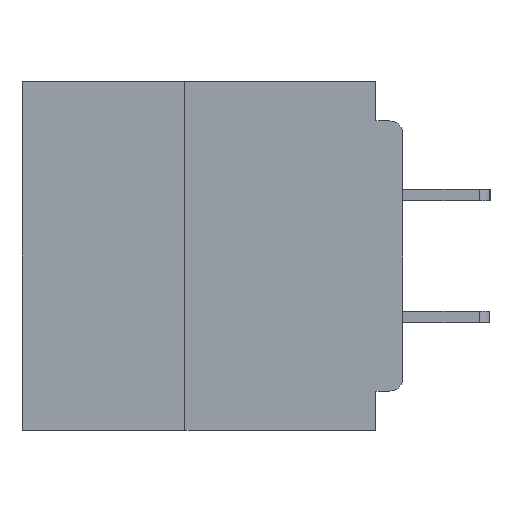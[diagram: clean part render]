
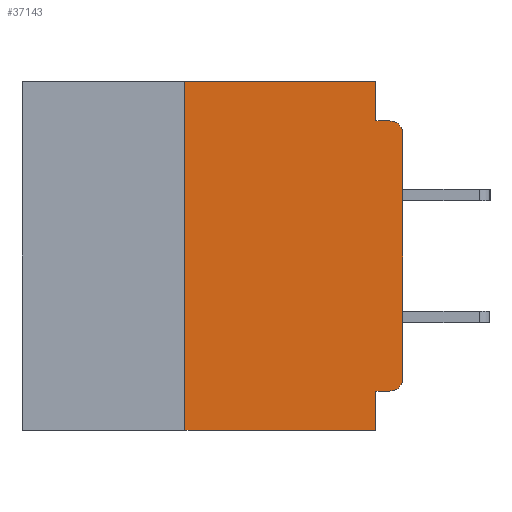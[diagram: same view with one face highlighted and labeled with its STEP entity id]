
A CAD part, left-side view. The second image highlights one B-rep face of the part: STEP entity #37143.
In plain terms, the highlighted planar face has unit normal (-1, 0, 0).
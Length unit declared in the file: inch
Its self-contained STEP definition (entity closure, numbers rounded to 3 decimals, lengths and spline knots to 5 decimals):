
#194 = CARTESIAN_POINT ( 'NONE',  ( 0., 0., -0.34 ) ) ;
#1139 = DIRECTION ( 'NONE',  ( 0., 0., 1. ) ) ;
#1416 = CARTESIAN_POINT ( 'NONE',  ( 0., 0.437, -0.4 ) ) ;
#1849 = DIRECTION ( 'NONE',  ( 0., 0., -1. ) ) ;
#1980 = CARTESIAN_POINT ( 'NONE',  ( 0., 0.031, -0.4 ) ) ;
#2558 = DIRECTION ( 'NONE',  ( 0., 0., -1. ) ) ;
#3075 = VERTEX_POINT ( 'NONE', #43019 ) ;
#3328 = EDGE_CURVE ( 'NONE', #17526, #16459, #58181, .T. ) ;
#5080 = AXIS2_PLACEMENT_3D ( 'NONE', #41207, #13744, #45778 ) ;
#6140 = LINE ( 'NONE', #47722, #52141 ) ;
#6951 = CARTESIAN_POINT ( 'NONE',  ( 0., 0.031, 0. ) ) ;
#7068 = PLANE ( 'NONE',  #7717 ) ;
#7717 = AXIS2_PLACEMENT_3D ( 'NONE', #52818, #30285, #2558 ) ;
#11805 = VECTOR ( 'NONE', #40488, 39.37008 ) ;
#12068 = DIRECTION ( 'NONE',  ( -1., 0., 0. ) ) ;
#13032 = VERTEX_POINT ( 'NONE', #49838 ) ;
#13688 = LINE ( 'NONE', #22514, #33827 ) ;
#13744 = DIRECTION ( 'NONE',  ( -1., 0., 0. ) ) ;
#14182 = EDGE_CURVE ( 'NONE', #31642, #31044, #6140, .T. ) ;
#15080 = VECTOR ( 'NONE', #39627, 39.37008 ) ;
#16413 = LINE ( 'NONE', #1416, #27245 ) ;
#16459 = VERTEX_POINT ( 'NONE', #194 ) ;
#17526 = VERTEX_POINT ( 'NONE', #19386 ) ;
#17550 = VERTEX_POINT ( 'NONE', #33222 ) ;
#17689 = CARTESIAN_POINT ( 'NONE',  ( 0., 0., 0. ) ) ;
#18527 = VECTOR ( 'NONE', #1139, 39.37008 ) ;
#19386 = CARTESIAN_POINT ( 'NONE',  ( 0., 0.015, -0.355 ) ) ;
#20598 = DIRECTION ( 'NONE',  ( 0., 1., 0. ) ) ;
#22514 = CARTESIAN_POINT ( 'NONE',  ( 0., 0.031, 0. ) ) ;
#23366 = EDGE_CURVE ( 'NONE', #48259, #13032, #50401, .T. ) ;
#23539 = CARTESIAN_POINT ( 'NONE',  ( 0., 0.25, 0. ) ) ;
#23822 = ORIENTED_EDGE ( 'NONE', *, *, #3328, .T. ) ;
#24265 = CARTESIAN_POINT ( 'NONE',  ( 0., 0.25, -0.4 ) ) ;
#24963 = ORIENTED_EDGE ( 'NONE', *, *, #56077, .F. ) ;
#25445 = VERTEX_POINT ( 'NONE', #23539 ) ;
#25500 = EDGE_CURVE ( 'NONE', #17550, #13032, #26323, .T. ) ;
#26066 = ORIENTED_EDGE ( 'NONE', *, *, #56413, .F. ) ;
#26150 = EDGE_CURVE ( 'NONE', #16459, #48259, #34818, .T. ) ;
#26323 = LINE ( 'NONE', #42097, #35615 ) ;
#27039 = ORIENTED_EDGE ( 'NONE', *, *, #53237, .F. ) ;
#27245 = VECTOR ( 'NONE', #51910, 39.37008 ) ;
#27362 = LINE ( 'NONE', #35068, #15080 ) ;
#28118 = CARTESIAN_POINT ( 'NONE',  ( 0., 0., -0.06 ) ) ;
#28963 = ORIENTED_EDGE ( 'NONE', *, *, #36351, .T. ) ;
#29972 = FACE_OUTER_BOUND ( 'NONE', #37342, .T. ) ;
#30285 = DIRECTION ( 'NONE',  ( 1., 0., 0. ) ) ;
#31044 = VERTEX_POINT ( 'NONE', #1980 ) ;
#31642 = VERTEX_POINT ( 'NONE', #51182 ) ;
#31909 = DIRECTION ( 'NONE',  ( 0., 0., -1. ) ) ;
#32464 = LINE ( 'NONE', #43373, #53875 ) ;
#33222 = CARTESIAN_POINT ( 'NONE',  ( 0., 0.031, -0.045 ) ) ;
#33699 = ORIENTED_EDGE ( 'NONE', *, *, #26150, .T. ) ;
#33827 = VECTOR ( 'NONE', #31909, 39.37008 ) ;
#34818 = LINE ( 'NONE', #17689, #11805 ) ;
#35068 = CARTESIAN_POINT ( 'NONE',  ( 0., 0.437, 0. ) ) ;
#35615 = VECTOR ( 'NONE', #46691, 39.37008 ) ;
#36351 = EDGE_CURVE ( 'NONE', #3075, #31044, #16413, .T. ) ;
#36957 = EDGE_CURVE ( 'NONE', #3075, #25445, #42836, .T. ) ;
#37143 = ADVANCED_FACE ( 'NONE', ( #29972 ), #7068, .F. ) ;
#37342 = EDGE_LOOP ( 'NONE', ( #33699, #42407, #50596, #24963, #26066, #41980, #28963, #55460, #27039, #23822 ) ) ;
#39539 = CARTESIAN_POINT ( 'NONE',  ( 0., 0.015, -0.06 ) ) ;
#39627 = DIRECTION ( 'NONE',  ( 0., -1., 0. ) ) ;
#40488 = DIRECTION ( 'NONE',  ( 0., 0., 1. ) ) ;
#41207 = CARTESIAN_POINT ( 'NONE',  ( 0., 0.015, -0.34 ) ) ;
#41980 = ORIENTED_EDGE ( 'NONE', *, *, #36957, .F. ) ;
#42097 = CARTESIAN_POINT ( 'NONE',  ( 0., 0., -0.045 ) ) ;
#42407 = ORIENTED_EDGE ( 'NONE', *, *, #23366, .T. ) ;
#42836 = LINE ( 'NONE', #24265, #18527 ) ;
#43019 = CARTESIAN_POINT ( 'NONE',  ( 0., 0.25, -0.4 ) ) ;
#43373 = CARTESIAN_POINT ( 'NONE',  ( 0., 0., -0.355 ) ) ;
#44133 = DIRECTION ( 'NONE',  ( 0., 0., -1. ) ) ;
#45778 = DIRECTION ( 'NONE',  ( 0., 0., -1. ) ) ;
#46691 = DIRECTION ( 'NONE',  ( 0., -1., 0. ) ) ;
#47722 = CARTESIAN_POINT ( 'NONE',  ( 0., 0.031, -0.4 ) ) ;
#48259 = VERTEX_POINT ( 'NONE', #28118 ) ;
#49838 = CARTESIAN_POINT ( 'NONE',  ( 0., 0.015, -0.045 ) ) ;
#50401 = CIRCLE ( 'NONE', #59419, 0.015 ) ;
#50596 = ORIENTED_EDGE ( 'NONE', *, *, #25500, .F. ) ;
#51182 = CARTESIAN_POINT ( 'NONE',  ( 0., 0.031, -0.355 ) ) ;
#51910 = DIRECTION ( 'NONE',  ( 0., -1., 0. ) ) ;
#52055 = VERTEX_POINT ( 'NONE', #6951 ) ;
#52141 = VECTOR ( 'NONE', #1849, 39.37008 ) ;
#52818 = CARTESIAN_POINT ( 'NONE',  ( 0., 0.437, 0. ) ) ;
#53237 = EDGE_CURVE ( 'NONE', #17526, #31642, #32464, .T. ) ;
#53875 = VECTOR ( 'NONE', #20598, 39.37008 ) ;
#55460 = ORIENTED_EDGE ( 'NONE', *, *, #14182, .F. ) ;
#56077 = EDGE_CURVE ( 'NONE', #52055, #17550, #13688, .T. ) ;
#56413 = EDGE_CURVE ( 'NONE', #25445, #52055, #27362, .T. ) ;
#58181 = CIRCLE ( 'NONE', #5080, 0.015 ) ;
#59419 = AXIS2_PLACEMENT_3D ( 'NONE', #39539, #12068, #44133 ) ;
